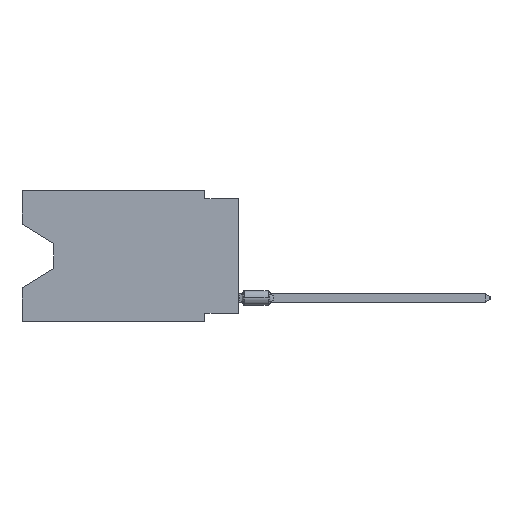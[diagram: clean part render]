
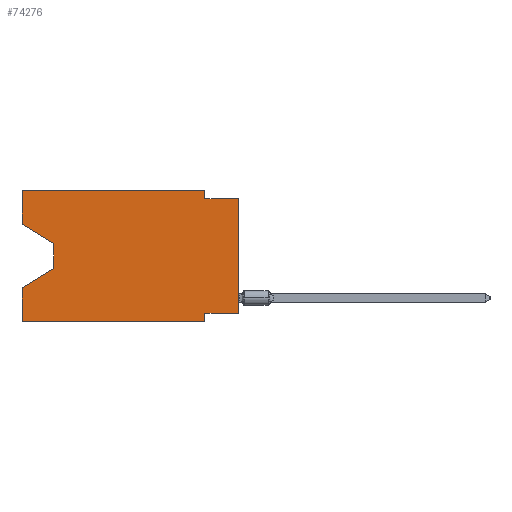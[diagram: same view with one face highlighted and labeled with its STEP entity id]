
A CAD part, left-side view. The second image highlights one B-rep face of the part: STEP entity #74276.
In plain terms, the highlighted planar face has unit normal (-1, 0, 0).
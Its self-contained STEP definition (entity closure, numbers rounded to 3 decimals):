
#56 = VECTOR ( 'NONE', #29850, 1000. ) ;
#948 = EDGE_CURVE ( 'NONE', #19450, #31965, #20918, .T. ) ;
#1863 = CARTESIAN_POINT ( 'NONE',  ( 0., 13.97, -4.013 ) ) ;
#2398 = VECTOR ( 'NONE', #28603, 1000. ) ;
#3801 = LINE ( 'NONE', #22374, #7528 ) ;
#3916 = LINE ( 'NONE', #64367, #35826 ) ;
#4852 = EDGE_CURVE ( 'NONE', #13023, #84554, #35474, .T. ) ;
#6632 = ORIENTED_EDGE ( 'NONE', *, *, #63956, .F. ) ;
#6711 = CARTESIAN_POINT ( 'NONE',  ( 0., 2.54, 0. ) ) ;
#7528 = VECTOR ( 'NONE', #82394, 1000. ) ;
#10785 = CARTESIAN_POINT ( 'NONE',  ( 0., 0., -9.271 ) ) ;
#11707 = VERTEX_POINT ( 'NONE', #36951 ) ;
#11715 = ORIENTED_EDGE ( 'NONE', *, *, #31244, .T. ) ;
#12224 = VERTEX_POINT ( 'NONE', #60137 ) ;
#12692 = ORIENTED_EDGE ( 'NONE', *, *, #29120, .T. ) ;
#13023 = VERTEX_POINT ( 'NONE', #82396 ) ;
#13910 = CARTESIAN_POINT ( 'NONE',  ( 0., 2.54, 0. ) ) ;
#14338 = DIRECTION ( 'NONE',  ( 0., 0., -1. ) ) ;
#17704 = CARTESIAN_POINT ( 'NONE',  ( 0., 16.383, 0. ) ) ;
#19450 = VERTEX_POINT ( 'NONE', #42224 ) ;
#20918 = LINE ( 'NONE', #74042, #72623 ) ;
#21754 = VERTEX_POINT ( 'NONE', #44682 ) ;
#21782 = DIRECTION ( 'NONE',  ( 0., -1., 0. ) ) ;
#22374 = CARTESIAN_POINT ( 'NONE',  ( 0., 0., 0. ) ) ;
#23712 = VERTEX_POINT ( 'NONE', #82541 ) ;
#24189 = VERTEX_POINT ( 'NONE', #6711 ) ;
#25021 = DIRECTION ( 'NONE',  ( 0., 0., -1. ) ) ;
#27235 = ORIENTED_EDGE ( 'NONE', *, *, #84655, .F. ) ;
#28603 = DIRECTION ( 'NONE',  ( 0., 0., -1. ) ) ;
#29120 = EDGE_CURVE ( 'NONE', #31965, #73619, #81736, .T. ) ;
#29850 = DIRECTION ( 'NONE',  ( 0., 0., -1. ) ) ;
#31244 = EDGE_CURVE ( 'NONE', #42456, #11707, #3801, .T. ) ;
#31965 = VERTEX_POINT ( 'NONE', #71329 ) ;
#33650 = ORIENTED_EDGE ( 'NONE', *, *, #52052, .F. ) ;
#35474 = LINE ( 'NONE', #36326, #56 ) ;
#35826 = VECTOR ( 'NONE', #43617, 1000. ) ;
#36326 = CARTESIAN_POINT ( 'NONE',  ( 0., 2.54, -9.906 ) ) ;
#36951 = CARTESIAN_POINT ( 'NONE',  ( 0., 0., -0.635 ) ) ;
#37570 = ORIENTED_EDGE ( 'NONE', *, *, #948, .T. ) ;
#37574 = CARTESIAN_POINT ( 'NONE',  ( 0., 16.383, 0. ) ) ;
#37959 = CARTESIAN_POINT ( 'NONE',  ( 0., 16.383, 0. ) ) ;
#37993 = VERTEX_POINT ( 'NONE', #79057 ) ;
#39822 = VECTOR ( 'NONE', #49647, 1000. ) ;
#39928 = EDGE_LOOP ( 'NONE', ( #37570, #12692, #67926, #33650, #64139, #41830, #27235, #11715, #44810, #66720, #6632, #82341 ) ) ;
#40278 = DIRECTION ( 'NONE',  ( 0., -1., 0. ) ) ;
#41319 = VECTOR ( 'NONE', #14338, 1000. ) ;
#41387 = VECTOR ( 'NONE', #76889, 1000. ) ;
#41830 = ORIENTED_EDGE ( 'NONE', *, *, #4852, .F. ) ;
#42224 = CARTESIAN_POINT ( 'NONE',  ( 0., 16.383, -2.546 ) ) ;
#42456 = VERTEX_POINT ( 'NONE', #10785 ) ;
#43617 = DIRECTION ( 'NONE',  ( 0., 1., 0. ) ) ;
#43775 = VECTOR ( 'NONE', #21782, 1000. ) ;
#44682 = CARTESIAN_POINT ( 'NONE',  ( 0., 16.383, 0. ) ) ;
#44810 = ORIENTED_EDGE ( 'NONE', *, *, #50461, .F. ) ;
#47989 = VECTOR ( 'NONE', #51659, 1000. ) ;
#49093 = LINE ( 'NONE', #75464, #47989 ) ;
#49647 = DIRECTION ( 'NONE',  ( 0., 0., 1. ) ) ;
#50461 = EDGE_CURVE ( 'NONE', #23712, #11707, #73129, .T. ) ;
#51659 = DIRECTION ( 'NONE',  ( 0., -1., 0. ) ) ;
#52052 = EDGE_CURVE ( 'NONE', #37993, #12224, #72003, .T. ) ;
#53079 = EDGE_CURVE ( 'NONE', #24189, #23712, #59676, .T. ) ;
#53300 = DIRECTION ( 'NONE',  ( 0., -0.855, -0.519 ) ) ;
#54600 = CARTESIAN_POINT ( 'NONE',  ( 0., 16.383, -9.906 ) ) ;
#56680 = VECTOR ( 'NONE', #40278, 1000. ) ;
#58235 = EDGE_CURVE ( 'NONE', #73619, #12224, #71834, .T. ) ;
#58266 = FACE_OUTER_BOUND ( 'NONE', #39928, .T. ) ;
#58685 = PLANE ( 'NONE',  #63828 ) ;
#59676 = LINE ( 'NONE', #13910, #41319 ) ;
#60137 = CARTESIAN_POINT ( 'NONE',  ( 0., 16.383, -7.36 ) ) ;
#61892 = VECTOR ( 'NONE', #78716, 1000. ) ;
#63828 = AXIS2_PLACEMENT_3D ( 'NONE', #37959, #78132, #25021 ) ;
#63956 = EDGE_CURVE ( 'NONE', #21754, #24189, #49093, .T. ) ;
#64139 = ORIENTED_EDGE ( 'NONE', *, *, #67973, .T. ) ;
#64367 = CARTESIAN_POINT ( 'NONE',  ( 0., 0., -9.271 ) ) ;
#66720 = ORIENTED_EDGE ( 'NONE', *, *, #53079, .F. ) ;
#67926 = ORIENTED_EDGE ( 'NONE', *, *, #58235, .T. ) ;
#67973 = EDGE_CURVE ( 'NONE', #37993, #84554, #68422, .T. ) ;
#68422 = LINE ( 'NONE', #54600, #43775 ) ;
#69135 = CARTESIAN_POINT ( 'NONE',  ( 0., 2.54, -9.906 ) ) ;
#71329 = CARTESIAN_POINT ( 'NONE',  ( 0., 13.97, -4.013 ) ) ;
#71834 = LINE ( 'NONE', #79136, #61892 ) ;
#72003 = LINE ( 'NONE', #37574, #41387 ) ;
#72623 = VECTOR ( 'NONE', #53300, 1000. ) ;
#73129 = LINE ( 'NONE', #74416, #56680 ) ;
#73619 = VERTEX_POINT ( 'NONE', #75885 ) ;
#74042 = CARTESIAN_POINT ( 'NONE',  ( 0., 16.383, -2.546 ) ) ;
#74276 = ADVANCED_FACE ( 'NONE', ( #58266 ), #58685, .F. ) ;
#74416 = CARTESIAN_POINT ( 'NONE',  ( 0., 0., -0.635 ) ) ;
#75464 = CARTESIAN_POINT ( 'NONE',  ( 0., 16.383, 0. ) ) ;
#75885 = CARTESIAN_POINT ( 'NONE',  ( 0., 13.97, -5.893 ) ) ;
#76875 = LINE ( 'NONE', #17704, #39822 ) ;
#76889 = DIRECTION ( 'NONE',  ( 0., 0., 1. ) ) ;
#78132 = DIRECTION ( 'NONE',  ( 1., 0., 0. ) ) ;
#78716 = DIRECTION ( 'NONE',  ( 0., 0.855, -0.519 ) ) ;
#79057 = CARTESIAN_POINT ( 'NONE',  ( 0., 16.383, -9.906 ) ) ;
#79136 = CARTESIAN_POINT ( 'NONE',  ( 0., 13.97, -5.893 ) ) ;
#81736 = LINE ( 'NONE', #1863, #2398 ) ;
#82341 = ORIENTED_EDGE ( 'NONE', *, *, #83459, .F. ) ;
#82394 = DIRECTION ( 'NONE',  ( 0., 0., 1. ) ) ;
#82396 = CARTESIAN_POINT ( 'NONE',  ( 0., 2.54, -9.271 ) ) ;
#82541 = CARTESIAN_POINT ( 'NONE',  ( 0., 2.54, -0.635 ) ) ;
#83459 = EDGE_CURVE ( 'NONE', #19450, #21754, #76875, .T. ) ;
#84554 = VERTEX_POINT ( 'NONE', #69135 ) ;
#84655 = EDGE_CURVE ( 'NONE', #42456, #13023, #3916, .T. ) ;
